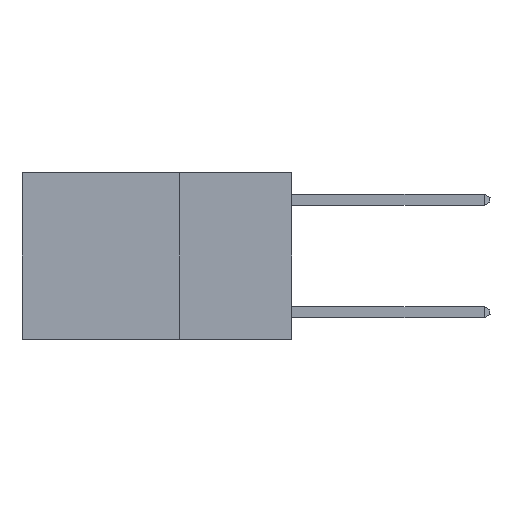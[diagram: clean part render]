
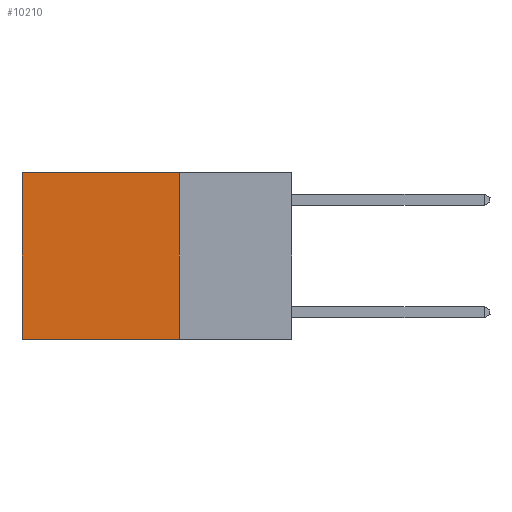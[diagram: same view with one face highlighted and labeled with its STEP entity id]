
A CAD part, left-side view. The second image highlights one B-rep face of the part: STEP entity #10210.
In plain terms, the highlighted planar face has unit normal (-1, 0, 0).
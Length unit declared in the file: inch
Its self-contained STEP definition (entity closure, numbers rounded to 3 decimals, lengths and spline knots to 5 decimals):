
#240 = CARTESIAN_POINT ( 'NONE',  ( 0.2625, 0.25, 0. ) ) ;
#336 = VECTOR ( 'NONE', #5605, 39.37008 ) ;
#750 = LINE ( 'NONE', #13999, #336 ) ;
#830 = VECTOR ( 'NONE', #7705, 39.37008 ) ;
#1304 = LINE ( 'NONE', #13296, #1876 ) ;
#1876 = VECTOR ( 'NONE', #12124, 39.37008 ) ;
#2001 = ORIENTED_EDGE ( 'NONE', *, *, #7948, .T. ) ;
#2303 = FACE_OUTER_BOUND ( 'NONE', #7991, .T. ) ;
#2378 = VERTEX_POINT ( 'NONE', #7320 ) ;
#3918 = LINE ( 'NONE', #6306, #830 ) ;
#4510 = EDGE_CURVE ( 'NONE', #7767, #2378, #750, .T. ) ;
#5605 = DIRECTION ( 'NONE',  ( 0., 1., 0. ) ) ;
#5643 = CARTESIAN_POINT ( 'NONE',  ( 0.2625, 0.25, 0. ) ) ;
#6220 = AXIS2_PLACEMENT_3D ( 'NONE', #240, #9943, #12161 ) ;
#6306 = CARTESIAN_POINT ( 'NONE',  ( 0.2625, 0.6, 0. ) ) ;
#7186 = DIRECTION ( 'NONE',  ( 0., 0., -1. ) ) ;
#7320 = CARTESIAN_POINT ( 'NONE',  ( 0.2625, 0.6, -0.37 ) ) ;
#7705 = DIRECTION ( 'NONE',  ( 0., 0., -1. ) ) ;
#7732 = EDGE_CURVE ( 'NONE', #10407, #7767, #8147, .T. ) ;
#7767 = VERTEX_POINT ( 'NONE', #9513 ) ;
#7948 = EDGE_CURVE ( 'NONE', #10407, #12831, #1304, .T. ) ;
#7991 = EDGE_LOOP ( 'NONE', ( #8899, #8854, #15522, #2001 ) ) ;
#8147 = LINE ( 'NONE', #15442, #9230 ) ;
#8854 = ORIENTED_EDGE ( 'NONE', *, *, #4510, .F. ) ;
#8899 = ORIENTED_EDGE ( 'NONE', *, *, #14779, .T. ) ;
#9230 = VECTOR ( 'NONE', #7186, 39.37008 ) ;
#9513 = CARTESIAN_POINT ( 'NONE',  ( 0.2625, 0.25, -0.37 ) ) ;
#9943 = DIRECTION ( 'NONE',  ( 1., 0., 0. ) ) ;
#10210 = ADVANCED_FACE ( 'NONE', ( #2303 ), #14605, .F. ) ;
#10407 = VERTEX_POINT ( 'NONE', #5643 ) ;
#12124 = DIRECTION ( 'NONE',  ( 0., 1., 0. ) ) ;
#12161 = DIRECTION ( 'NONE',  ( 0., 0., -1. ) ) ;
#12831 = VERTEX_POINT ( 'NONE', #15430 ) ;
#13296 = CARTESIAN_POINT ( 'NONE',  ( 0.2625, 0.25, 0. ) ) ;
#13999 = CARTESIAN_POINT ( 'NONE',  ( 0.2625, 0.25, -0.37 ) ) ;
#14605 = PLANE ( 'NONE',  #6220 ) ;
#14779 = EDGE_CURVE ( 'NONE', #12831, #2378, #3918, .T. ) ;
#15430 = CARTESIAN_POINT ( 'NONE',  ( 0.2625, 0.6, 0. ) ) ;
#15442 = CARTESIAN_POINT ( 'NONE',  ( 0.2625, 0.25, 0. ) ) ;
#15522 = ORIENTED_EDGE ( 'NONE', *, *, #7732, .F. ) ;
